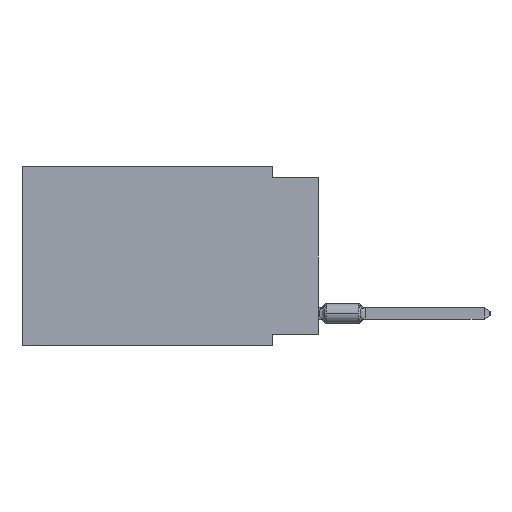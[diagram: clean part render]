
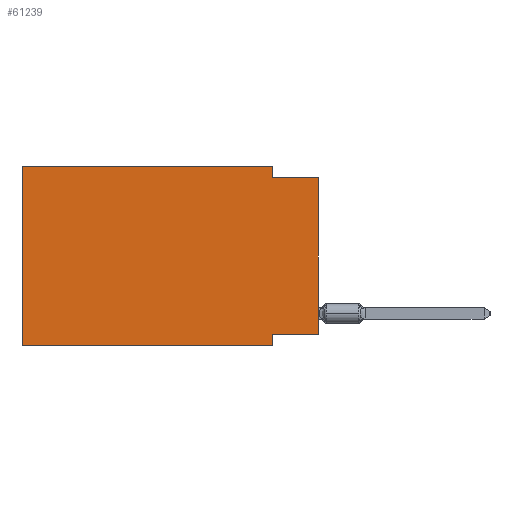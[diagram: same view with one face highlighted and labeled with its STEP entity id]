
A CAD part, left-side view. The second image highlights one B-rep face of the part: STEP entity #61239.
In plain terms, the highlighted planar face has unit normal (-1, 0, 0).
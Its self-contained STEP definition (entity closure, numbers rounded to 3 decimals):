
#617 = CARTESIAN_POINT ( 'NONE',  ( 0., 0., -0.635 ) ) ;
#1144 = CARTESIAN_POINT ( 'NONE',  ( 0., 0., -9.271 ) ) ;
#3036 = DIRECTION ( 'NONE',  ( 1., 0., 0. ) ) ;
#3632 = EDGE_LOOP ( 'NONE', ( #66191, #48644, #69230, #68541, #83270, #37605, #41930, #47509 ) ) ;
#8133 = CARTESIAN_POINT ( 'NONE',  ( 0., 0., -9.271 ) ) ;
#11593 = LINE ( 'NONE', #62633, #45253 ) ;
#16744 = VECTOR ( 'NONE', #33821, 1000. ) ;
#16930 = CARTESIAN_POINT ( 'NONE',  ( 0., 2.54, -9.906 ) ) ;
#17029 = FACE_OUTER_BOUND ( 'NONE', #3632, .T. ) ;
#18613 = CARTESIAN_POINT ( 'NONE',  ( 0., 16.383, 0. ) ) ;
#19334 = LINE ( 'NONE', #71628, #41360 ) ;
#20567 = CARTESIAN_POINT ( 'NONE',  ( 0., 0., -0.635 ) ) ;
#21638 = EDGE_CURVE ( 'NONE', #70567, #56103, #39643, .T. ) ;
#27854 = LINE ( 'NONE', #46564, #34086 ) ;
#32836 = CARTESIAN_POINT ( 'NONE',  ( 0., 2.54, -9.271 ) ) ;
#33821 = DIRECTION ( 'NONE',  ( 0., 1., 0. ) ) ;
#34086 = VECTOR ( 'NONE', #53800, 1000. ) ;
#34532 = EDGE_CURVE ( 'NONE', #34631, #61753, #43130, .T. ) ;
#34631 = VERTEX_POINT ( 'NONE', #64802 ) ;
#36148 = CARTESIAN_POINT ( 'NONE',  ( 0., 16.383, 0. ) ) ;
#36749 = CARTESIAN_POINT ( 'NONE',  ( 0., 16.383, 0. ) ) ;
#37605 = ORIENTED_EDGE ( 'NONE', *, *, #62271, .T. ) ;
#38540 = VECTOR ( 'NONE', #39228, 1000. ) ;
#39228 = DIRECTION ( 'NONE',  ( 0., 0., -1. ) ) ;
#39643 = LINE ( 'NONE', #77907, #38540 ) ;
#41360 = VECTOR ( 'NONE', #65664, 1000. ) ;
#41930 = ORIENTED_EDGE ( 'NONE', *, *, #79221, .F. ) ;
#42578 = VERTEX_POINT ( 'NONE', #32836 ) ;
#43130 = LINE ( 'NONE', #36749, #78114 ) ;
#44275 = CARTESIAN_POINT ( 'NONE',  ( 0., 0., 0. ) ) ;
#45253 = VECTOR ( 'NONE', #55820, 1000. ) ;
#45510 = DIRECTION ( 'NONE',  ( 0., 0., 1. ) ) ;
#46463 = CARTESIAN_POINT ( 'NONE',  ( 0., 2.54, 0. ) ) ;
#46564 = CARTESIAN_POINT ( 'NONE',  ( 0., 16.383, 0. ) ) ;
#46916 = LINE ( 'NONE', #20567, #56013 ) ;
#47509 = ORIENTED_EDGE ( 'NONE', *, *, #59101, .F. ) ;
#48644 = ORIENTED_EDGE ( 'NONE', *, *, #74129, .F. ) ;
#50368 = CARTESIAN_POINT ( 'NONE',  ( 0., 2.54, -0.635 ) ) ;
#53159 = EDGE_CURVE ( 'NONE', #71097, #72972, #77813, .T. ) ;
#53800 = DIRECTION ( 'NONE',  ( 0., -1., 0. ) ) ;
#55028 = AXIS2_PLACEMENT_3D ( 'NONE', #36148, #3036, #75691 ) ;
#55820 = DIRECTION ( 'NONE',  ( 0., 0., -1. ) ) ;
#56013 = VECTOR ( 'NONE', #78800, 1000. ) ;
#56103 = VERTEX_POINT ( 'NONE', #50368 ) ;
#58364 = VERTEX_POINT ( 'NONE', #16930 ) ;
#59101 = EDGE_CURVE ( 'NONE', #71097, #42578, #79296, .T. ) ;
#61239 = ADVANCED_FACE ( 'NONE', ( #17029 ), #74003, .F. ) ;
#61753 = VERTEX_POINT ( 'NONE', #18613 ) ;
#62271 = EDGE_CURVE ( 'NONE', #34631, #58364, #19334, .T. ) ;
#62633 = CARTESIAN_POINT ( 'NONE',  ( 0., 2.54, -9.906 ) ) ;
#62661 = VECTOR ( 'NONE', #45510, 1000. ) ;
#62702 = DIRECTION ( 'NONE',  ( 0., 0., 1. ) ) ;
#64802 = CARTESIAN_POINT ( 'NONE',  ( 0., 16.383, -9.906 ) ) ;
#65664 = DIRECTION ( 'NONE',  ( 0., -1., 0. ) ) ;
#66191 = ORIENTED_EDGE ( 'NONE', *, *, #53159, .T. ) ;
#68541 = ORIENTED_EDGE ( 'NONE', *, *, #72515, .F. ) ;
#69230 = ORIENTED_EDGE ( 'NONE', *, *, #21638, .F. ) ;
#70567 = VERTEX_POINT ( 'NONE', #46463 ) ;
#71097 = VERTEX_POINT ( 'NONE', #8133 ) ;
#71628 = CARTESIAN_POINT ( 'NONE',  ( 0., 16.383, -9.906 ) ) ;
#72515 = EDGE_CURVE ( 'NONE', #61753, #70567, #27854, .T. ) ;
#72972 = VERTEX_POINT ( 'NONE', #617 ) ;
#74003 = PLANE ( 'NONE',  #55028 ) ;
#74129 = EDGE_CURVE ( 'NONE', #56103, #72972, #46916, .T. ) ;
#75691 = DIRECTION ( 'NONE',  ( 0., 0., -1. ) ) ;
#77813 = LINE ( 'NONE', #44275, #62661 ) ;
#77907 = CARTESIAN_POINT ( 'NONE',  ( 0., 2.54, 0. ) ) ;
#78114 = VECTOR ( 'NONE', #62702, 1000. ) ;
#78800 = DIRECTION ( 'NONE',  ( 0., -1., 0. ) ) ;
#79221 = EDGE_CURVE ( 'NONE', #42578, #58364, #11593, .T. ) ;
#79296 = LINE ( 'NONE', #1144, #16744 ) ;
#83270 = ORIENTED_EDGE ( 'NONE', *, *, #34532, .F. ) ;
